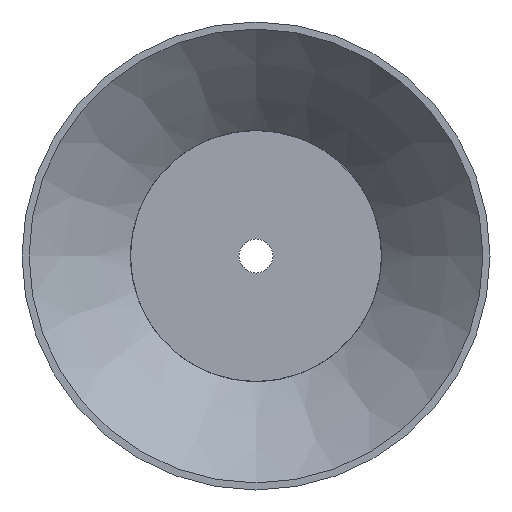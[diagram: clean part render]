
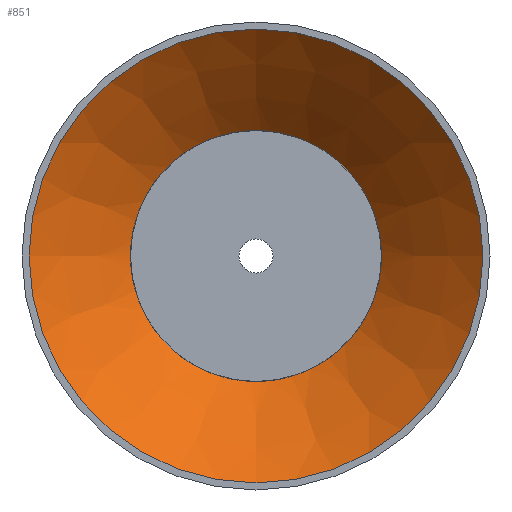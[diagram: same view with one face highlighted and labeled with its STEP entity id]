
A CAD part, front view. The second image highlights one B-rep face of the part: STEP entity #851.
In plain terms, the highlighted conical face has half-angle 44.868 degrees and reference radius 31.488 mm.
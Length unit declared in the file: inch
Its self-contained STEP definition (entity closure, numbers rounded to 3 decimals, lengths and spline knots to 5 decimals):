
#126=FACE_OUTER_BOUND('',#166,.T.);
#166=EDGE_LOOP('',(#559,#560,#561,#562,#563,#564,#565,#566,#567,#568,#569,
#570,#571,#572,#573,#574,#575,#576,#577,#578,#579));
#209=(
BOUNDED_CURVE()
B_SPLINE_CURVE(2,(#1136,#1137,#1138),.UNSPECIFIED.,.F.,.F.)
B_SPLINE_CURVE_WITH_KNOTS((3,3),(0.,0.02339),.UNSPECIFIED.)
CURVE()
GEOMETRIC_REPRESENTATION_ITEM()
RATIONAL_B_SPLINE_CURVE((1.,1.,1.))
REPRESENTATION_ITEM('')
);
#210=(
BOUNDED_CURVE()
B_SPLINE_CURVE(2,(#1142,#1143,#1144),.UNSPECIFIED.,.F.,.F.)
B_SPLINE_CURVE_WITH_KNOTS((3,3),(0.96217,0.98555),
 .UNSPECIFIED.)
CURVE()
GEOMETRIC_REPRESENTATION_ITEM()
RATIONAL_B_SPLINE_CURVE((1.,1.,1.))
REPRESENTATION_ITEM('')
);
#211=(
BOUNDED_CURVE()
B_SPLINE_CURVE(2,(#1148,#1149,#1150),.UNSPECIFIED.,.F.,.F.)
B_SPLINE_CURVE_WITH_KNOTS((3,3),(0.,0.02339),.UNSPECIFIED.)
CURVE()
GEOMETRIC_REPRESENTATION_ITEM()
RATIONAL_B_SPLINE_CURVE((1.,1.,1.))
REPRESENTATION_ITEM('')
);
#212=(
BOUNDED_CURVE()
B_SPLINE_CURVE(2,(#1154,#1155,#1156),.UNSPECIFIED.,.F.,.F.)
B_SPLINE_CURVE_WITH_KNOTS((3,3),(0.96221,0.98559),
 .UNSPECIFIED.)
CURVE()
GEOMETRIC_REPRESENTATION_ITEM()
RATIONAL_B_SPLINE_CURVE((1.,1.,1.))
REPRESENTATION_ITEM('')
);
#213=(
BOUNDED_CURVE()
B_SPLINE_CURVE(2,(#1160,#1161,#1162),.UNSPECIFIED.,.F.,.F.)
B_SPLINE_CURVE_WITH_KNOTS((3,3),(0.,0.02339),.UNSPECIFIED.)
CURVE()
GEOMETRIC_REPRESENTATION_ITEM()
RATIONAL_B_SPLINE_CURVE((1.,1.,1.))
REPRESENTATION_ITEM('')
);
#214=(
BOUNDED_CURVE()
B_SPLINE_CURVE(2,(#1166,#1167,#1168),.UNSPECIFIED.,.F.,.F.)
B_SPLINE_CURVE_WITH_KNOTS((3,3),(0.96233,0.98572),
 .UNSPECIFIED.)
CURVE()
GEOMETRIC_REPRESENTATION_ITEM()
RATIONAL_B_SPLINE_CURVE((1.,1.,1.))
REPRESENTATION_ITEM('')
);
#215=(
BOUNDED_CURVE()
B_SPLINE_CURVE(2,(#1172,#1173,#1174),.UNSPECIFIED.,.F.,.F.)
B_SPLINE_CURVE_WITH_KNOTS((3,3),(0.,0.02339),.UNSPECIFIED.)
CURVE()
GEOMETRIC_REPRESENTATION_ITEM()
RATIONAL_B_SPLINE_CURVE((1.,1.,1.))
REPRESENTATION_ITEM('')
);
#216=(
BOUNDED_CURVE()
B_SPLINE_CURVE(2,(#1178,#1179,#1180),.UNSPECIFIED.,.F.,.F.)
B_SPLINE_CURVE_WITH_KNOTS((3,3),(0.96221,0.9856),
 .UNSPECIFIED.)
CURVE()
GEOMETRIC_REPRESENTATION_ITEM()
RATIONAL_B_SPLINE_CURVE((1.,1.,1.))
REPRESENTATION_ITEM('')
);
#218=LINE('',#1132,#248);
#248=VECTOR('',#974,1.23967);
#278=CIRCLE('',#906,1.6);
#279=CIRCLE('',#907,0.885);
#280=CIRCLE('',#908,0.87933);
#281=CIRCLE('',#909,0.885);
#282=CIRCLE('',#910,0.87933);
#283=CIRCLE('',#911,0.885);
#284=CIRCLE('',#912,0.87933);
#285=CIRCLE('',#913,0.885);
#286=CIRCLE('',#914,0.87933);
#287=CIRCLE('',#915,0.885);
#288=CIRCLE('',#916,1.6);
#314=VERTEX_POINT('',#1128);
#315=VERTEX_POINT('',#1129);
#316=VERTEX_POINT('',#1131);
#317=VERTEX_POINT('',#1133);
#318=VERTEX_POINT('',#1135);
#319=VERTEX_POINT('',#1139);
#320=VERTEX_POINT('',#1141);
#321=VERTEX_POINT('',#1145);
#322=VERTEX_POINT('',#1147);
#323=VERTEX_POINT('',#1151);
#324=VERTEX_POINT('',#1153);
#325=VERTEX_POINT('',#1157);
#326=VERTEX_POINT('',#1159);
#327=VERTEX_POINT('',#1163);
#328=VERTEX_POINT('',#1165);
#329=VERTEX_POINT('',#1169);
#330=VERTEX_POINT('',#1171);
#331=VERTEX_POINT('',#1175);
#332=VERTEX_POINT('',#1177);
#414=EDGE_CURVE('',#314,#315,#278,.T.);
#415=EDGE_CURVE('',#315,#316,#218,.T.);
#416=EDGE_CURVE('',#317,#316,#279,.T.);
#417=EDGE_CURVE('',#318,#317,#209,.T.);
#418=EDGE_CURVE('',#319,#318,#280,.T.);
#419=EDGE_CURVE('',#320,#319,#210,.T.);
#420=EDGE_CURVE('',#321,#320,#281,.T.);
#421=EDGE_CURVE('',#322,#321,#211,.T.);
#422=EDGE_CURVE('',#323,#322,#282,.T.);
#423=EDGE_CURVE('',#324,#323,#212,.T.);
#424=EDGE_CURVE('',#325,#324,#283,.T.);
#425=EDGE_CURVE('',#326,#325,#213,.T.);
#426=EDGE_CURVE('',#327,#326,#284,.T.);
#427=EDGE_CURVE('',#328,#327,#214,.T.);
#428=EDGE_CURVE('',#329,#328,#285,.T.);
#429=EDGE_CURVE('',#330,#329,#215,.T.);
#430=EDGE_CURVE('',#331,#330,#286,.T.);
#431=EDGE_CURVE('',#332,#331,#216,.T.);
#432=EDGE_CURVE('',#316,#332,#287,.T.);
#433=EDGE_CURVE('',#315,#314,#288,.T.);
#559=ORIENTED_EDGE('',*,*,#414,.T.);
#560=ORIENTED_EDGE('',*,*,#415,.T.);
#561=ORIENTED_EDGE('',*,*,#416,.F.);
#562=ORIENTED_EDGE('',*,*,#417,.F.);
#563=ORIENTED_EDGE('',*,*,#418,.F.);
#564=ORIENTED_EDGE('',*,*,#419,.F.);
#565=ORIENTED_EDGE('',*,*,#420,.F.);
#566=ORIENTED_EDGE('',*,*,#421,.F.);
#567=ORIENTED_EDGE('',*,*,#422,.F.);
#568=ORIENTED_EDGE('',*,*,#423,.F.);
#569=ORIENTED_EDGE('',*,*,#424,.F.);
#570=ORIENTED_EDGE('',*,*,#425,.F.);
#571=ORIENTED_EDGE('',*,*,#426,.F.);
#572=ORIENTED_EDGE('',*,*,#427,.F.);
#573=ORIENTED_EDGE('',*,*,#428,.F.);
#574=ORIENTED_EDGE('',*,*,#429,.F.);
#575=ORIENTED_EDGE('',*,*,#430,.F.);
#576=ORIENTED_EDGE('',*,*,#431,.F.);
#577=ORIENTED_EDGE('',*,*,#432,.F.);
#578=ORIENTED_EDGE('',*,*,#415,.F.);
#579=ORIENTED_EDGE('',*,*,#433,.T.);
#849=CONICAL_SURFACE('',#905,1.23967,0.783);
#851=ADVANCED_FACE('',(#126),#849,.F.);
#905=AXIS2_PLACEMENT_3D('',#1127,#970,#971);
#906=AXIS2_PLACEMENT_3D('',#1130,#972,#973);
#907=AXIS2_PLACEMENT_3D('',#1134,#975,#976);
#908=AXIS2_PLACEMENT_3D('',#1140,#977,#978);
#909=AXIS2_PLACEMENT_3D('',#1146,#979,#980);
#910=AXIS2_PLACEMENT_3D('',#1152,#981,#982);
#911=AXIS2_PLACEMENT_3D('',#1158,#983,#984);
#912=AXIS2_PLACEMENT_3D('',#1164,#985,#986);
#913=AXIS2_PLACEMENT_3D('',#1170,#987,#988);
#914=AXIS2_PLACEMENT_3D('',#1176,#989,#990);
#915=AXIS2_PLACEMENT_3D('',#1181,#991,#992);
#916=AXIS2_PLACEMENT_3D('',#1182,#993,#994);
#970=DIRECTION('center_axis',(0.,-1.,0.));
#971=DIRECTION('ref_axis',(1.,0.,0.));
#972=DIRECTION('center_axis',(0.,-1.,0.));
#973=DIRECTION('ref_axis',(1.,0.,0.));
#974=DIRECTION('',(0.705,0.709,0.));
#975=DIRECTION('center_axis',(0.,-1.,0.));
#976=DIRECTION('ref_axis',(1.,0.,0.));
#977=DIRECTION('center_axis',(0.,-1.,0.));
#978=DIRECTION('ref_axis',(1.,0.,0.));
#979=DIRECTION('center_axis',(0.,-1.,0.));
#980=DIRECTION('ref_axis',(1.,0.,0.));
#981=DIRECTION('center_axis',(0.,-1.,0.));
#982=DIRECTION('ref_axis',(1.,0.,0.));
#983=DIRECTION('center_axis',(0.,-1.,0.));
#984=DIRECTION('ref_axis',(1.,0.,0.));
#985=DIRECTION('center_axis',(0.,-1.,0.));
#986=DIRECTION('ref_axis',(1.,0.,0.));
#987=DIRECTION('center_axis',(0.,-1.,0.));
#988=DIRECTION('ref_axis',(1.,0.,0.));
#989=DIRECTION('center_axis',(0.,-1.,0.));
#990=DIRECTION('ref_axis',(1.,0.,0.));
#991=DIRECTION('center_axis',(0.,-1.,0.));
#992=DIRECTION('ref_axis',(1.,0.,0.));
#993=DIRECTION('center_axis',(0.,-1.,0.));
#994=DIRECTION('ref_axis',(1.,0.,0.));
#1127=CARTESIAN_POINT('Origin',(0.,0.362,0.));
#1128=CARTESIAN_POINT('',(1.6,0.,0.));
#1129=CARTESIAN_POINT('',(-1.6,0.,0.));
#1130=CARTESIAN_POINT('Origin',(0.,0.,
0.));
#1131=CARTESIAN_POINT('',(-0.885,0.7183,0.));
#1132=CARTESIAN_POINT('',(-1.23967,0.362,0.));
#1133=CARTESIAN_POINT('',(-0.87933,0.7183,0.09998));
#1134=CARTESIAN_POINT('Origin',(0.,0.7183,0.));
#1135=CARTESIAN_POINT('',(-0.87363,0.724,0.09998));
#1136=CARTESIAN_POINT('Ctrl Pts',(-0.87363,0.724,0.09998));
#1137=CARTESIAN_POINT('Ctrl Pts',(-0.87647,0.72116,
0.09998));
#1138=CARTESIAN_POINT('Ctrl Pts',(-0.87933,0.7183,
0.09998));
#1139=CARTESIAN_POINT('',(-0.10007,0.724,0.87362));
#1140=CARTESIAN_POINT('Origin',(0.,0.724,0.));
#1141=CARTESIAN_POINT('',(-0.10007,0.7183,0.87932));
#1142=CARTESIAN_POINT('Ctrl Pts',(-0.10007,0.7183,
0.87932));
#1143=CARTESIAN_POINT('Ctrl Pts',(-0.10007,0.72116,
0.87646));
#1144=CARTESIAN_POINT('Ctrl Pts',(-0.10007,0.724,0.87362));
#1145=CARTESIAN_POINT('',(0.09984,0.7183,0.87935));
#1146=CARTESIAN_POINT('Origin',(0.,0.7183,0.));
#1147=CARTESIAN_POINT('',(0.09984,0.724,0.87364));
#1148=CARTESIAN_POINT('Ctrl Pts',(0.09984,0.724,0.87364));
#1149=CARTESIAN_POINT('Ctrl Pts',(0.09984,0.72116,
0.87649));
#1150=CARTESIAN_POINT('Ctrl Pts',(0.09984,0.7183,
0.87935));
#1151=CARTESIAN_POINT('',(0.87362,0.724,0.10001));
#1152=CARTESIAN_POINT('Origin',(0.,0.724,0.));
#1153=CARTESIAN_POINT('',(0.87933,0.7183,0.10001));
#1154=CARTESIAN_POINT('Ctrl Pts',(0.87933,0.7183,0.10001));
#1155=CARTESIAN_POINT('Ctrl Pts',(0.87647,0.72116,0.10001));
#1156=CARTESIAN_POINT('Ctrl Pts',(0.87362,0.724,0.10001));
#1157=CARTESIAN_POINT('',(0.87933,0.7183,-0.10006));
#1158=CARTESIAN_POINT('Origin',(0.,0.7183,0.));
#1159=CARTESIAN_POINT('',(0.87362,0.724,-0.10006));
#1160=CARTESIAN_POINT('Ctrl Pts',(0.87362,0.724,-0.10006));
#1161=CARTESIAN_POINT('Ctrl Pts',(0.87646,0.72116,-0.10006));
#1162=CARTESIAN_POINT('Ctrl Pts',(0.87933,0.7183,-0.10006));
#1163=CARTESIAN_POINT('',(0.09984,0.724,-0.87364));
#1164=CARTESIAN_POINT('Origin',(0.,0.724,0.));
#1165=CARTESIAN_POINT('',(0.09984,0.7183,-0.87935));
#1166=CARTESIAN_POINT('Ctrl Pts',(0.09984,0.7183,
-0.87935));
#1167=CARTESIAN_POINT('Ctrl Pts',(0.09984,0.72116,-0.87649));
#1168=CARTESIAN_POINT('Ctrl Pts',(0.09984,0.724,-0.87364));
#1169=CARTESIAN_POINT('',(-0.09997,0.7183,-0.87934));
#1170=CARTESIAN_POINT('Origin',(0.,0.7183,0.));
#1171=CARTESIAN_POINT('',(-0.09997,0.724,-0.87363));
#1172=CARTESIAN_POINT('Ctrl Pts',(-0.09997,0.724,-0.87363));
#1173=CARTESIAN_POINT('Ctrl Pts',(-0.09997,0.72116,
-0.87647));
#1174=CARTESIAN_POINT('Ctrl Pts',(-0.09997,0.7183,
-0.87934));
#1175=CARTESIAN_POINT('',(-0.87363,0.724,-0.1));
#1176=CARTESIAN_POINT('Origin',(0.,0.724,0.));
#1177=CARTESIAN_POINT('',(-0.87933,0.7183,-0.1));
#1178=CARTESIAN_POINT('Ctrl Pts',(-0.87933,0.7183,
-0.1));
#1179=CARTESIAN_POINT('Ctrl Pts',(-0.87647,0.72116,
-0.1));
#1180=CARTESIAN_POINT('Ctrl Pts',(-0.87363,0.724,-0.1));
#1181=CARTESIAN_POINT('Origin',(0.,0.7183,0.));
#1182=CARTESIAN_POINT('Origin',(0.,0.,
0.));
